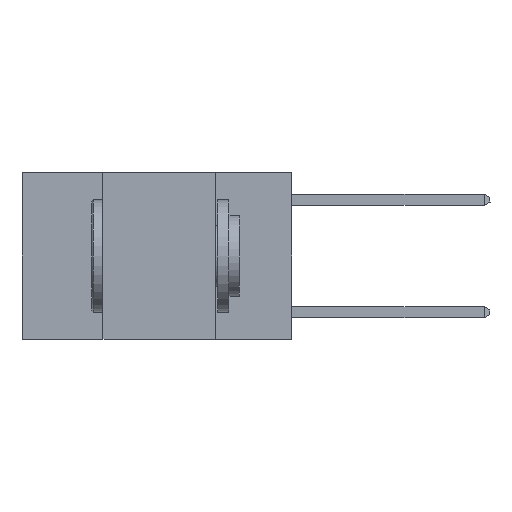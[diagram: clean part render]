
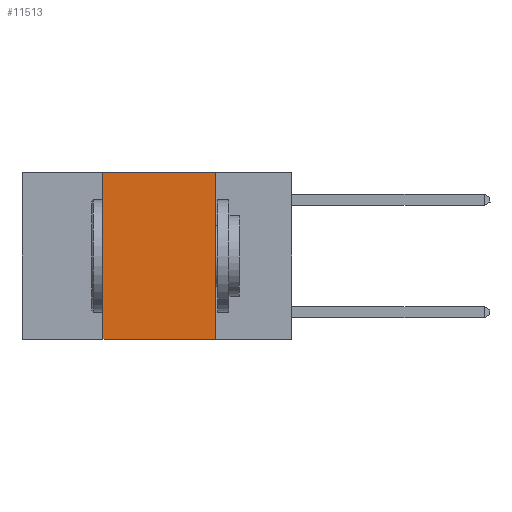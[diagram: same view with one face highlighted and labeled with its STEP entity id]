
A CAD part, left-side view. The second image highlights one B-rep face of the part: STEP entity #11513.
In plain terms, the highlighted planar face has unit normal (-1, 0, 0).
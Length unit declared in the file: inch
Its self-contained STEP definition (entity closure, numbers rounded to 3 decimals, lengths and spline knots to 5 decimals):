
#689 = ORIENTED_EDGE ( 'NONE', *, *, #8097, .F. ) ;
#1544 = DIRECTION ( 'NONE',  ( 1., 0., 0. ) ) ;
#1729 = ORIENTED_EDGE ( 'NONE', *, *, #17336, .T. ) ;
#2378 = LINE ( 'NONE', #26083, #12549 ) ;
#4725 = CARTESIAN_POINT ( 'NONE',  ( 0., 0.42, 0. ) ) ;
#5348 = AXIS2_PLACEMENT_3D ( 'NONE', #25053, #1544, #16683 ) ;
#5855 = CARTESIAN_POINT ( 'NONE',  ( 0., 0.17, 0. ) ) ;
#6917 = DIRECTION ( 'NONE',  ( 0., 0., 1. ) ) ;
#7424 = VECTOR ( 'NONE', #24973, 39.37008 ) ;
#7885 = CARTESIAN_POINT ( 'NONE',  ( 0., 0.6, 0. ) ) ;
#8097 = EDGE_CURVE ( 'NONE', #20543, #14415, #13619, .T. ) ;
#8199 = VECTOR ( 'NONE', #6917, 39.37008 ) ;
#11203 = DIRECTION ( 'NONE',  ( 0., -1., 0. ) ) ;
#11513 = ADVANCED_FACE ( 'NONE', ( #20138 ), #18719, .F. ) ;
#11877 = ORIENTED_EDGE ( 'NONE', *, *, #23994, .F. ) ;
#12192 = ORIENTED_EDGE ( 'NONE', *, *, #19651, .F. ) ;
#12549 = VECTOR ( 'NONE', #11203, 39.37008 ) ;
#12719 = CARTESIAN_POINT ( 'NONE',  ( 0., 0.17, 0. ) ) ;
#13619 = LINE ( 'NONE', #12719, #18682 ) ;
#14415 = VERTEX_POINT ( 'NONE', #25769 ) ;
#14888 = DIRECTION ( 'NONE',  ( 0., 0., -1. ) ) ;
#16683 = DIRECTION ( 'NONE',  ( 0., 0., -1. ) ) ;
#17336 = EDGE_CURVE ( 'NONE', #23061, #14415, #2378, .T. ) ;
#18682 = VECTOR ( 'NONE', #14888, 39.37008 ) ;
#18719 = PLANE ( 'NONE',  #5348 ) ;
#19313 = VERTEX_POINT ( 'NONE', #21783 ) ;
#19651 = EDGE_CURVE ( 'NONE', #19313, #20543, #23814, .T. ) ;
#20138 = FACE_OUTER_BOUND ( 'NONE', #26181, .T. ) ;
#20543 = VERTEX_POINT ( 'NONE', #5855 ) ;
#21783 = CARTESIAN_POINT ( 'NONE',  ( 0., 0.42, 0. ) ) ;
#23061 = VERTEX_POINT ( 'NONE', #26933 ) ;
#23814 = LINE ( 'NONE', #7885, #7424 ) ;
#23994 = EDGE_CURVE ( 'NONE', #23061, #19313, #25247, .T. ) ;
#24973 = DIRECTION ( 'NONE',  ( 0., -1., 0. ) ) ;
#25053 = CARTESIAN_POINT ( 'NONE',  ( 0., 0.6, 0. ) ) ;
#25247 = LINE ( 'NONE', #4725, #8199 ) ;
#25769 = CARTESIAN_POINT ( 'NONE',  ( 0., 0.17, -0.37 ) ) ;
#26083 = CARTESIAN_POINT ( 'NONE',  ( 0., 0.6, -0.37 ) ) ;
#26181 = EDGE_LOOP ( 'NONE', ( #689, #12192, #11877, #1729 ) ) ;
#26933 = CARTESIAN_POINT ( 'NONE',  ( 0., 0.42, -0.37 ) ) ;
